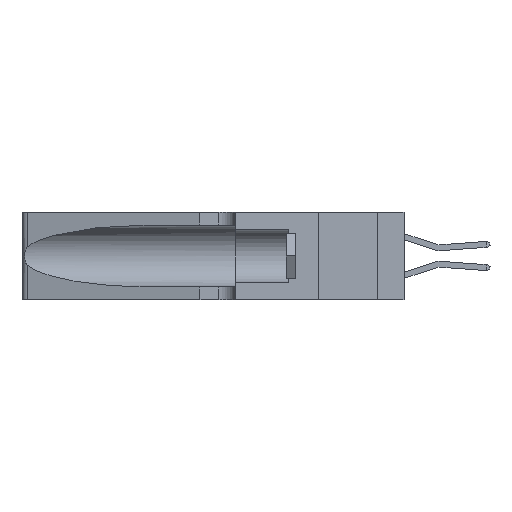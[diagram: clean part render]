
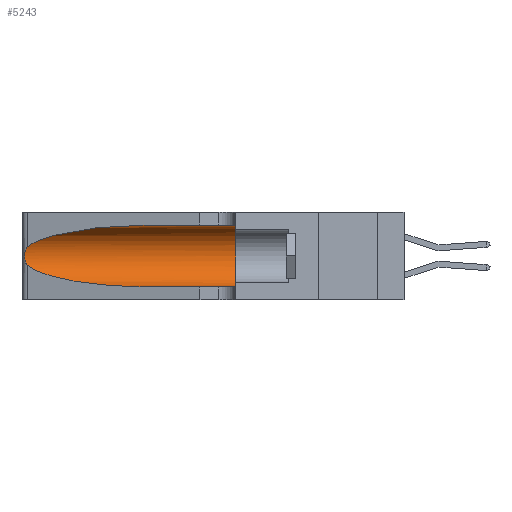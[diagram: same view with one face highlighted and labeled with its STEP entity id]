
A CAD part, left-side view. The second image highlights one B-rep face of the part: STEP entity #5243.
In plain terms, the highlighted cylindrical face has radius 3.308 mm (diameter 6.617 mm), a partial arc.
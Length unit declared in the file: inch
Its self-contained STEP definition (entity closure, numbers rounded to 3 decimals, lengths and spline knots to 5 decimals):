
#31 = CARTESIAN_POINT ( 'NONE',  ( 0.25854, 1.2359, 0.20912 ) ) ;
#1106 =( BOUNDED_CURVE ( )  B_SPLINE_CURVE ( 3, ( #10487, #20507, #29510, #13757 ),
 .UNSPECIFIED., .F., .T. ) 
 B_SPLINE_CURVE_WITH_KNOTS ( ( 4, 4 ),
 ( 3.44316, 4.71239 ),
 .UNSPECIFIED. ) 
 CURVE ( )  GEOMETRIC_REPRESENTATION_ITEM ( )  RATIONAL_B_SPLINE_CURVE ( ( 1., 0.87, 0.87, 1. ) ) 
 REPRESENTATION_ITEM ( '' )  );
#1213 = CARTESIAN_POINT ( 'NONE',  ( 0.1305, 1.61858, 0.05475 ) ) ;
#1551 = CARTESIAN_POINT ( 'NONE',  ( 0.18966, 0.96281, 0.31525 ) ) ;
#1850 = EDGE_CURVE ( 'NONE', #38346, #38997, #21190, .T. ) ;
#2690 = ORIENTED_EDGE ( 'NONE', *, *, #33607, .F. ) ;
#3017 = VERTEX_POINT ( 'NONE', #27620 ) ;
#4845 = ORIENTED_EDGE ( 'NONE', *, *, #30385, .T. ) ;
#5243 = ADVANCED_FACE ( 'NONE', ( #5443 ), #16696, .F. ) ;
#5443 = FACE_OUTER_BOUND ( 'NONE', #34315, .T. ) ;
#6173 = CARTESIAN_POINT ( 'NONE',  ( 0.25555, 1.22994, 0.2215 ) ) ;
#6314 = CARTESIAN_POINT ( 'NONE',  ( 0.25487, 1.22718, 0.22369 ) ) ;
#6818 = EDGE_CURVE ( 'NONE', #35286, #38997, #23003, .T. ) ;
#7217 = DIRECTION ( 'NONE',  ( 0., -1., 0. ) ) ;
#9129 = VECTOR ( 'NONE', #39970, 39.37008 ) ;
#9617 = VERTEX_POINT ( 'NONE', #24092 ) ;
#10282 = DIRECTION ( 'NONE',  ( 0., 1., 0. ) ) ;
#10487 = CARTESIAN_POINT ( 'NONE',  ( 0.25487, 1.22718, 0.14631 ) ) ;
#12040 = CARTESIAN_POINT ( 'NONE',  ( 0.25789, 1.23486, 0.15765 ) ) ;
#12143 = AXIS2_PLACEMENT_3D ( 'NONE', #26099, #34897, #38572 ) ;
#12464 = CARTESIAN_POINT ( 'NONE',  ( 0.25856, 1.23593, 0.16098 ) ) ;
#13515 = LINE ( 'NONE', #18028, #9129 ) ;
#13757 = CARTESIAN_POINT ( 'NONE',  ( 0.1305, 0.72297, 0.05475 ) ) ;
#13970 = CARTESIAN_POINT ( 'NONE',  ( 0.2373, 1.15595, 0.28018 ) ) ;
#14393 = ORIENTED_EDGE ( 'NONE', *, *, #6818, .F. ) ;
#16102 = AXIS2_PLACEMENT_3D ( 'NONE', #35240, #10282, #28905 ) ;
#16696 = CYLINDRICAL_SURFACE ( 'NONE', #12143, 0.13025 ) ;
#16897 = B_SPLINE_CURVE_WITH_KNOTS ( 'NONE', 3,
 ( #6314, #6173, #30825, #24671, #31, #21939, #28198, #27684, #37572, #12464, #12040, #18769, #37165, #18356 ),
 .UNSPECIFIED., .F., .F.,
 ( 4, 2, 2, 2, 2, 2, 4 ),
 ( 0., 0.00027, 0.00053, 0.00107, 0.0016, 0.00187, 0.00214 ),
 .UNSPECIFIED. ) ;
#17162 = CARTESIAN_POINT ( 'NONE',  ( 0.1305, 0.35, 0.05475 ) ) ;
#18028 = CARTESIAN_POINT ( 'NONE',  ( 0.1305, 1.61858, 0.31525 ) ) ;
#18356 = CARTESIAN_POINT ( 'NONE',  ( 0.25487, 1.22718, 0.14631 ) ) ;
#18769 = CARTESIAN_POINT ( 'NONE',  ( 0.25639, 1.23186, 0.15144 ) ) ;
#20507 = CARTESIAN_POINT ( 'NONE',  ( 0.2373, 1.15595, 0.08982 ) ) ;
#21058 = EDGE_CURVE ( 'NONE', #3017, #40118, #25946, .T. ) ;
#21190 = LINE ( 'NONE', #1213, #33934 ) ;
#21664 = ORIENTED_EDGE ( 'NONE', *, *, #1850, .T. ) ;
#21939 = CARTESIAN_POINT ( 'NONE',  ( 0.26018, 1.23835, 0.19895 ) ) ;
#23003 = CIRCLE ( 'NONE', #16102, 0.13025 ) ;
#23713 = CARTESIAN_POINT ( 'NONE',  ( 0.1305, 0.72297, 0.31525 ) ) ;
#23824 = ORIENTED_EDGE ( 'NONE', *, *, #29404, .T. ) ;
#24092 = CARTESIAN_POINT ( 'NONE',  ( 0.25487, 1.22718, 0.14631 ) ) ;
#24671 = CARTESIAN_POINT ( 'NONE',  ( 0.25787, 1.23484, 0.2124 ) ) ;
#25946 =( BOUNDED_CURVE ( )  B_SPLINE_CURVE ( 3, ( #23713, #1551, #13970, #29996 ),
 .UNSPECIFIED., .F., .F. ) 
 B_SPLINE_CURVE_WITH_KNOTS ( ( 4, 4 ),
 ( 1.5708, 2.84003 ),
 .UNSPECIFIED. ) 
 CURVE ( )  GEOMETRIC_REPRESENTATION_ITEM ( )  RATIONAL_B_SPLINE_CURVE ( ( 1., 0.87, 0.87, 1. ) ) 
 REPRESENTATION_ITEM ( '' )  );
#26099 = CARTESIAN_POINT ( 'NONE',  ( 0.1305, 1.61858, 0.185 ) ) ;
#26416 = CARTESIAN_POINT ( 'NONE',  ( 0.1305, 0.72297, 0.05475 ) ) ;
#27620 = CARTESIAN_POINT ( 'NONE',  ( 0.1305, 0.72297, 0.31525 ) ) ;
#27684 = CARTESIAN_POINT ( 'NONE',  ( 0.26075, 1.23896, 0.178 ) ) ;
#28198 = CARTESIAN_POINT ( 'NONE',  ( 0.26075, 1.23896, 0.19203 ) ) ;
#28905 = DIRECTION ( 'NONE',  ( 0., 0., 1. ) ) ;
#29404 = EDGE_CURVE ( 'NONE', #9617, #38346, #1106, .T. ) ;
#29510 = CARTESIAN_POINT ( 'NONE',  ( 0.18966, 0.96281, 0.05475 ) ) ;
#29996 = CARTESIAN_POINT ( 'NONE',  ( 0.25487, 1.22718, 0.22369 ) ) ;
#30385 = EDGE_CURVE ( 'NONE', #40118, #9617, #16897, .T. ) ;
#30825 = CARTESIAN_POINT ( 'NONE',  ( 0.25639, 1.23184, 0.21858 ) ) ;
#33095 = CARTESIAN_POINT ( 'NONE',  ( 0.1305, 0.35, 0.31525 ) ) ;
#33607 = EDGE_CURVE ( 'NONE', #3017, #35286, #13515, .T. ) ;
#33934 = VECTOR ( 'NONE', #7217, 39.37008 ) ;
#34315 = EDGE_LOOP ( 'NONE', ( #37221, #4845, #23824, #21664, #14393, #2690 ) ) ;
#34897 = DIRECTION ( 'NONE',  ( 0., -1., 0. ) ) ;
#35240 = CARTESIAN_POINT ( 'NONE',  ( 0.1305, 0.35, 0.185 ) ) ;
#35286 = VERTEX_POINT ( 'NONE', #33095 ) ;
#37165 = CARTESIAN_POINT ( 'NONE',  ( 0.25555, 1.22993, 0.14849 ) ) ;
#37221 = ORIENTED_EDGE ( 'NONE', *, *, #21058, .T. ) ;
#37572 = CARTESIAN_POINT ( 'NONE',  ( 0.26017, 1.23833, 0.17102 ) ) ;
#38308 = CARTESIAN_POINT ( 'NONE',  ( 0.25487, 1.22718, 0.22369 ) ) ;
#38346 = VERTEX_POINT ( 'NONE', #26416 ) ;
#38572 = DIRECTION ( 'NONE',  ( 0., 0., -1. ) ) ;
#38997 = VERTEX_POINT ( 'NONE', #17162 ) ;
#39970 = DIRECTION ( 'NONE',  ( 0., -1., 0. ) ) ;
#40118 = VERTEX_POINT ( 'NONE', #38308 ) ;
